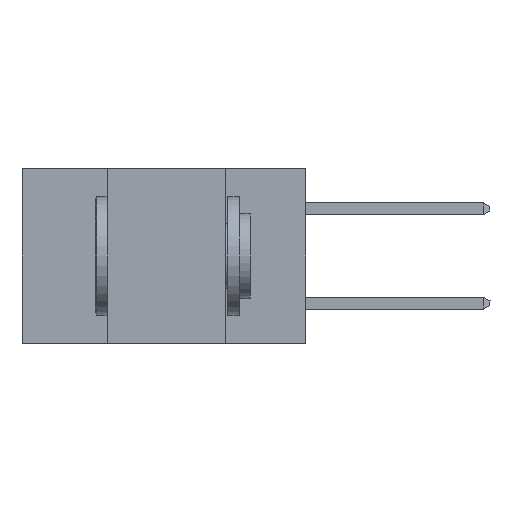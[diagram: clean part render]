
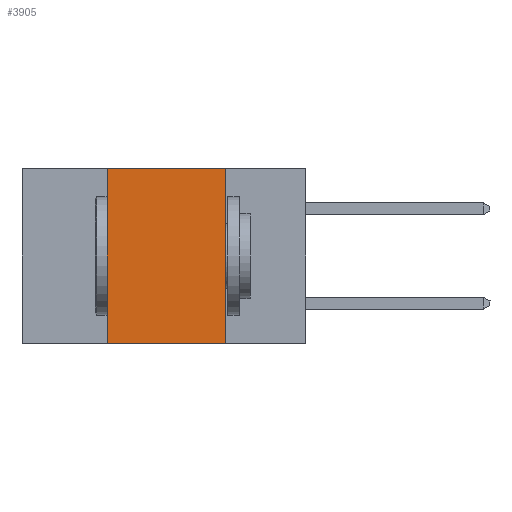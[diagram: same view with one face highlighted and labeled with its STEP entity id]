
A CAD part, left-side view. The second image highlights one B-rep face of the part: STEP entity #3905.
In plain terms, the highlighted planar face has unit normal (-1, 0, 0).
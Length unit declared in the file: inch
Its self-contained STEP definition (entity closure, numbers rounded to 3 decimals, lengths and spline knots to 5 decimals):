
#148 = EDGE_LOOP ( 'NONE', ( #5921, #4139, #5727, #10006 ) ) ;
#716 = CARTESIAN_POINT ( 'NONE',  ( 0., 0.6, 0. ) ) ;
#759 = CARTESIAN_POINT ( 'NONE',  ( 0., 0.6, 0. ) ) ;
#1805 = AXIS2_PLACEMENT_3D ( 'NONE', #759, #7213, #6187 ) ;
#1985 = VERTEX_POINT ( 'NONE', #2722 ) ;
#2072 = CARTESIAN_POINT ( 'NONE',  ( 0., 0.17, 0. ) ) ;
#2722 = CARTESIAN_POINT ( 'NONE',  ( 0., 0.42, 0. ) ) ;
#3312 = DIRECTION ( 'NONE',  ( 0., -1., 0. ) ) ;
#3521 = PLANE ( 'NONE',  #1805 ) ;
#3905 = ADVANCED_FACE ( 'NONE', ( #10316 ), #3521, .F. ) ;
#3958 = EDGE_CURVE ( 'NONE', #1985, #7825, #11788, .T. ) ;
#4041 = VERTEX_POINT ( 'NONE', #9132 ) ;
#4139 = ORIENTED_EDGE ( 'NONE', *, *, #3958, .F. ) ;
#4925 = DIRECTION ( 'NONE',  ( 0., 0., -1. ) ) ;
#5229 = CARTESIAN_POINT ( 'NONE',  ( 0., 0.17, 0. ) ) ;
#5727 = ORIENTED_EDGE ( 'NONE', *, *, #11817, .F. ) ;
#5921 = ORIENTED_EDGE ( 'NONE', *, *, #11535, .F. ) ;
#6044 = VECTOR ( 'NONE', #4925, 39.37008 ) ;
#6057 = VECTOR ( 'NONE', #11604, 39.37008 ) ;
#6097 = VERTEX_POINT ( 'NONE', #7612 ) ;
#6187 = DIRECTION ( 'NONE',  ( 0., 0., -1. ) ) ;
#6811 = EDGE_CURVE ( 'NONE', #6097, #4041, #10415, .T. ) ;
#7136 = DIRECTION ( 'NONE',  ( 0., -1., 0. ) ) ;
#7213 = DIRECTION ( 'NONE',  ( 1., 0., 0. ) ) ;
#7612 = CARTESIAN_POINT ( 'NONE',  ( 0., 0.42, -0.37 ) ) ;
#7825 = VERTEX_POINT ( 'NONE', #5229 ) ;
#8578 = LINE ( 'NONE', #8778, #6057 ) ;
#8765 = CARTESIAN_POINT ( 'NONE',  ( 0., 0.6, -0.37 ) ) ;
#8778 = CARTESIAN_POINT ( 'NONE',  ( 0., 0.42, 0. ) ) ;
#9132 = CARTESIAN_POINT ( 'NONE',  ( 0., 0.17, -0.37 ) ) ;
#10006 = ORIENTED_EDGE ( 'NONE', *, *, #6811, .T. ) ;
#10316 = FACE_OUTER_BOUND ( 'NONE', #148, .T. ) ;
#10415 = LINE ( 'NONE', #8765, #11592 ) ;
#11163 = LINE ( 'NONE', #2072, #6044 ) ;
#11496 = VECTOR ( 'NONE', #7136, 39.37008 ) ;
#11535 = EDGE_CURVE ( 'NONE', #7825, #4041, #11163, .T. ) ;
#11592 = VECTOR ( 'NONE', #3312, 39.37008 ) ;
#11604 = DIRECTION ( 'NONE',  ( 0., 0., 1. ) ) ;
#11788 = LINE ( 'NONE', #716, #11496 ) ;
#11817 = EDGE_CURVE ( 'NONE', #6097, #1985, #8578, .T. ) ;
